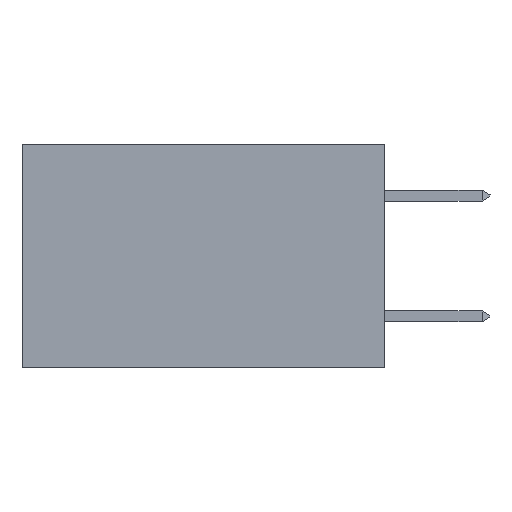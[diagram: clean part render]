
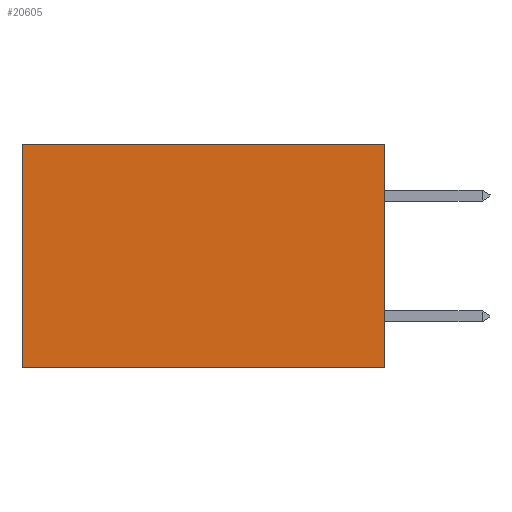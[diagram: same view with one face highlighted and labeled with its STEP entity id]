
A CAD part, left-side view. The second image highlights one B-rep face of the part: STEP entity #20605.
In plain terms, the highlighted planar face has unit normal (-1, 0, 0).
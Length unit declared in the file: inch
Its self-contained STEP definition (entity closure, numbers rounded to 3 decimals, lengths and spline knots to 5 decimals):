
#1599 = VECTOR ( 'NONE', #18640, 39.37008 ) ;
#1601 = DIRECTION ( 'NONE',  ( 1., 0., 0. ) ) ;
#2299 = DIRECTION ( 'NONE',  ( 0., 0., -1. ) ) ;
#3188 = VECTOR ( 'NONE', #17557, 39.37008 ) ;
#3407 = DIRECTION ( 'NONE',  ( 0., 1., 0. ) ) ;
#3663 = VERTEX_POINT ( 'NONE', #12906 ) ;
#3687 = ORIENTED_EDGE ( 'NONE', *, *, #9268, .F. ) ;
#3969 = CARTESIAN_POINT ( 'NONE',  ( 0.2875, 0., -0.37 ) ) ;
#4422 = AXIS2_PLACEMENT_3D ( 'NONE', #21056, #1601, #13160 ) ;
#4433 = CARTESIAN_POINT ( 'NONE',  ( 0.2875, 0.6, 0. ) ) ;
#4850 = LINE ( 'NONE', #16460, #8751 ) ;
#5327 = LINE ( 'NONE', #12195, #9727 ) ;
#5466 = EDGE_LOOP ( 'NONE', ( #9284, #3687, #8632, #7639 ) ) ;
#7012 = EDGE_CURVE ( 'NONE', #3663, #12966, #5327, .T. ) ;
#7639 = ORIENTED_EDGE ( 'NONE', *, *, #17516, .T. ) ;
#8434 = EDGE_CURVE ( 'NONE', #8928, #9423, #11986, .T. ) ;
#8632 = ORIENTED_EDGE ( 'NONE', *, *, #7012, .F. ) ;
#8751 = VECTOR ( 'NONE', #3407, 39.37008 ) ;
#8928 = VERTEX_POINT ( 'NONE', #14344 ) ;
#9268 = EDGE_CURVE ( 'NONE', #12966, #9423, #10349, .T. ) ;
#9284 = ORIENTED_EDGE ( 'NONE', *, *, #8434, .T. ) ;
#9423 = VERTEX_POINT ( 'NONE', #14261 ) ;
#9727 = VECTOR ( 'NONE', #2299, 39.37008 ) ;
#9836 = PLANE ( 'NONE',  #4422 ) ;
#10349 = LINE ( 'NONE', #3969, #1599 ) ;
#11986 = LINE ( 'NONE', #4433, #3188 ) ;
#12195 = CARTESIAN_POINT ( 'NONE',  ( 0.2875, 0., 0. ) ) ;
#12906 = CARTESIAN_POINT ( 'NONE',  ( 0.2875, 0., 0. ) ) ;
#12966 = VERTEX_POINT ( 'NONE', #18597 ) ;
#13160 = DIRECTION ( 'NONE',  ( 0., 0., -1. ) ) ;
#14261 = CARTESIAN_POINT ( 'NONE',  ( 0.2875, 0.6, -0.37 ) ) ;
#14344 = CARTESIAN_POINT ( 'NONE',  ( 0.2875, 0.6, 0. ) ) ;
#15760 = FACE_OUTER_BOUND ( 'NONE', #5466, .T. ) ;
#16460 = CARTESIAN_POINT ( 'NONE',  ( 0.2875, 0., 0. ) ) ;
#17516 = EDGE_CURVE ( 'NONE', #3663, #8928, #4850, .T. ) ;
#17557 = DIRECTION ( 'NONE',  ( 0., 0., -1. ) ) ;
#18597 = CARTESIAN_POINT ( 'NONE',  ( 0.2875, 0., -0.37 ) ) ;
#18640 = DIRECTION ( 'NONE',  ( 0., 1., 0. ) ) ;
#20605 = ADVANCED_FACE ( 'NONE', ( #15760 ), #9836, .F. ) ;
#21056 = CARTESIAN_POINT ( 'NONE',  ( 0.2875, 0., 0. ) ) ;
